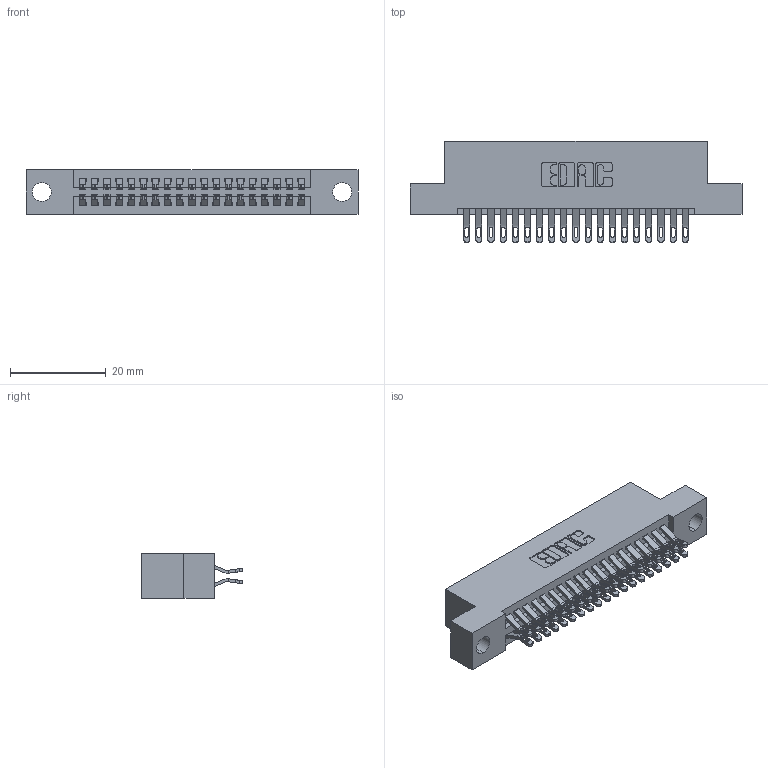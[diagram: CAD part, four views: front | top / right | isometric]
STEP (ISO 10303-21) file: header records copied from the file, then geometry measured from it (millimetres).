
FILE_DESCRIPTION (( 'STEP AP203' ), '1' );
FILE_NAME ('395-038-555-204.STEP', '2021-06-16T21:36:05', ( '' ), ( '' ), 'SwSTEP 2.0', 'SolidWorks 2020', '' );
FILE_SCHEMA (( 'CONFIG_CONTROL_DESIGN' ));
Length unit declared in the file: inch
Products named in the file (3): 345 Part_Flush Mounting Lugs - 0.156 Dia-TI; 395-038-555-204; 345-292-001_555 Tail
Assembly tree (39 placements, depth 2):
  395-038-555-204
    345 Part_Flush Mounting Lugs - 0.156 Dia-TI
    345-292-001_555 Tail  x38
Bounding box: 69.47 x 21.13 x 9.4 mm (x, y, z)
Volume: 6539.1 mm3; surface area: 9455.3 mm2
Topology: 39 solids, 39 shells, 2268 faces, 7103 edges, 4734 vertices
Faces by surface type: plane 1272, cylinder 996
Entity records: 18749 total; most frequent: CARTESIAN_POINT 3204, ORIENTED_EDGE 3106, DIRECTION 2821, EDGE_CURVE 1553, VECTOR 1325, LINE 1325, VERTEX_POINT 1034, AXIS2_PLACEMENT_3D 748
